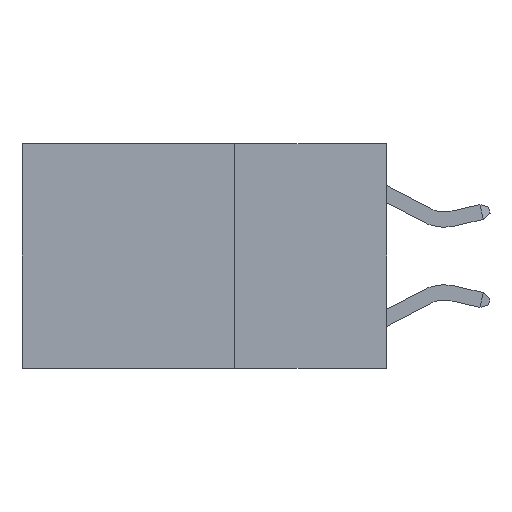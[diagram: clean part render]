
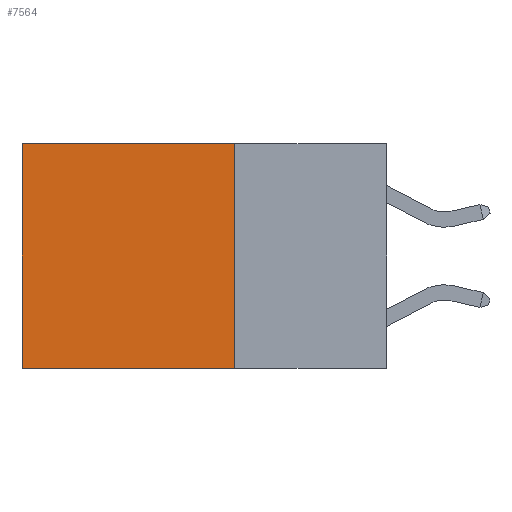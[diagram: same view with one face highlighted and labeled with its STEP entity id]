
A CAD part, left-side view. The second image highlights one B-rep face of the part: STEP entity #7564.
In plain terms, the highlighted planar face has unit normal (-1, 0, 0).
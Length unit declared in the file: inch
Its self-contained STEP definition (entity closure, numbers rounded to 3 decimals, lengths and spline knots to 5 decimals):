
#325 = EDGE_CURVE ( 'NONE', #5412, #8858, #14295, .T. ) ;
#939 = CARTESIAN_POINT ( 'NONE',  ( 0.2625, 0.6, -0.37 ) ) ;
#1585 = VECTOR ( 'NONE', #14168, 39.37008 ) ;
#2938 = FACE_OUTER_BOUND ( 'NONE', #27905, .T. ) ;
#3143 = ORIENTED_EDGE ( 'NONE', *, *, #12630, .T. ) ;
#3995 = DIRECTION ( 'NONE',  ( 0., 0., -1. ) ) ;
#4305 = DIRECTION ( 'NONE',  ( 1., 0., 0. ) ) ;
#4400 = CARTESIAN_POINT ( 'NONE',  ( 0.2625, 0.25, 0. ) ) ;
#5252 = EDGE_CURVE ( 'NONE', #13226, #24160, #29295, .T. ) ;
#5412 = VERTEX_POINT ( 'NONE', #8224 ) ;
#6517 = PLANE ( 'NONE',  #25496 ) ;
#7564 = ADVANCED_FACE ( 'NONE', ( #2938 ), #6517, .F. ) ;
#8224 = CARTESIAN_POINT ( 'NONE',  ( 0.2625, 0.6, 0. ) ) ;
#8631 = CARTESIAN_POINT ( 'NONE',  ( 0.2625, 0.6, 0. ) ) ;
#8858 = VERTEX_POINT ( 'NONE', #939 ) ;
#11646 = VECTOR ( 'NONE', #20903, 39.37008 ) ;
#12630 = EDGE_CURVE ( 'NONE', #13226, #5412, #17756, .T. ) ;
#13226 = VERTEX_POINT ( 'NONE', #4400 ) ;
#13802 = LINE ( 'NONE', #18797, #1585 ) ;
#14168 = DIRECTION ( 'NONE',  ( 0., 1., 0. ) ) ;
#14295 = LINE ( 'NONE', #8631, #21861 ) ;
#17756 = LINE ( 'NONE', #27754, #11646 ) ;
#18054 = CARTESIAN_POINT ( 'NONE',  ( 0.2625, 0.25, 0. ) ) ;
#18797 = CARTESIAN_POINT ( 'NONE',  ( 0.2625, 0.25, -0.37 ) ) ;
#20372 = DIRECTION ( 'NONE',  ( 0., 0., -1. ) ) ;
#20802 = ORIENTED_EDGE ( 'NONE', *, *, #24706, .F. ) ;
#20903 = DIRECTION ( 'NONE',  ( 0., 1., 0. ) ) ;
#21861 = VECTOR ( 'NONE', #3995, 39.37008 ) ;
#23360 = DIRECTION ( 'NONE',  ( 0., 0., -1. ) ) ;
#23830 = ORIENTED_EDGE ( 'NONE', *, *, #325, .T. ) ;
#24160 = VERTEX_POINT ( 'NONE', #28682 ) ;
#24237 = ORIENTED_EDGE ( 'NONE', *, *, #5252, .F. ) ;
#24706 = EDGE_CURVE ( 'NONE', #24160, #8858, #13802, .T. ) ;
#25496 = AXIS2_PLACEMENT_3D ( 'NONE', #18054, #4305, #20372 ) ;
#27754 = CARTESIAN_POINT ( 'NONE',  ( 0.2625, 0.25, 0. ) ) ;
#27886 = CARTESIAN_POINT ( 'NONE',  ( 0.2625, 0.25, 0. ) ) ;
#27905 = EDGE_LOOP ( 'NONE', ( #23830, #20802, #24237, #3143 ) ) ;
#28588 = VECTOR ( 'NONE', #23360, 39.37008 ) ;
#28682 = CARTESIAN_POINT ( 'NONE',  ( 0.2625, 0.25, -0.37 ) ) ;
#29295 = LINE ( 'NONE', #27886, #28588 ) ;
